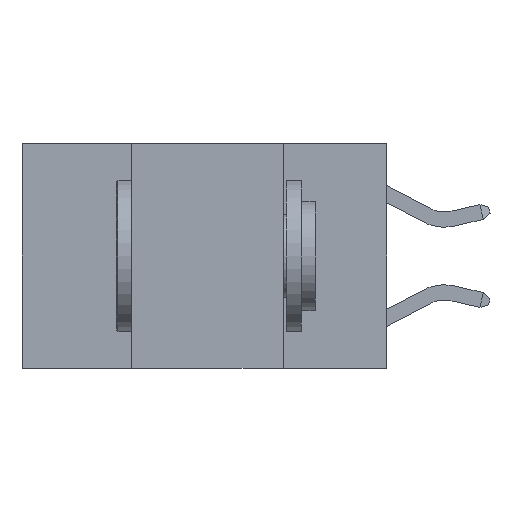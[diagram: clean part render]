
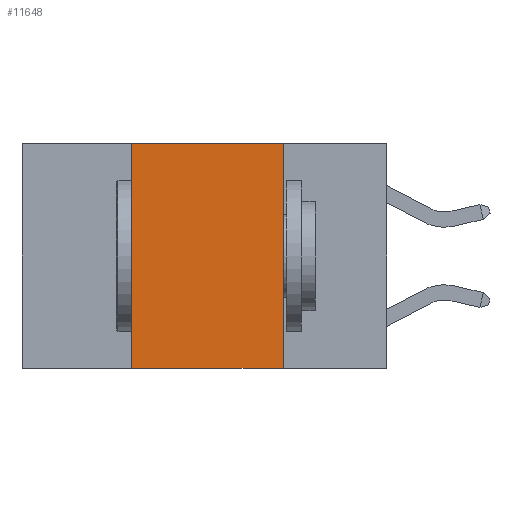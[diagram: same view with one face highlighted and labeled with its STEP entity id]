
A CAD part, left-side view. The second image highlights one B-rep face of the part: STEP entity #11648.
In plain terms, the highlighted planar face has unit normal (-1, 0, 0).
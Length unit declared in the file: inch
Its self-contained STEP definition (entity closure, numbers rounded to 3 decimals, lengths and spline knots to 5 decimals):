
#240 = AXIS2_PLACEMENT_3D ( 'NONE', #6873, #6803, #13682 ) ;
#523 = EDGE_CURVE ( 'NONE', #5476, #7634, #9982, .T. ) ;
#686 = CARTESIAN_POINT ( 'NONE',  ( 0., 0.42, 0. ) ) ;
#1471 = FACE_OUTER_BOUND ( 'NONE', #8806, .T. ) ;
#2809 = DIRECTION ( 'NONE',  ( 0., 0., -1. ) ) ;
#2942 = DIRECTION ( 'NONE',  ( 0., -1., 0. ) ) ;
#3037 = LINE ( 'NONE', #10507, #8568 ) ;
#3136 = ORIENTED_EDGE ( 'NONE', *, *, #13306, .F. ) ;
#3306 = CARTESIAN_POINT ( 'NONE',  ( 0., 0.42, 0. ) ) ;
#3372 = ORIENTED_EDGE ( 'NONE', *, *, #5863, .F. ) ;
#3624 = VECTOR ( 'NONE', #10059, 39.37008 ) ;
#3645 = CARTESIAN_POINT ( 'NONE',  ( 0., 0.42, -0.37 ) ) ;
#4118 = CARTESIAN_POINT ( 'NONE',  ( 0., 0.17, 0. ) ) ;
#4455 = VECTOR ( 'NONE', #12003, 39.37008 ) ;
#5221 = LINE ( 'NONE', #7504, #5804 ) ;
#5476 = VERTEX_POINT ( 'NONE', #686 ) ;
#5502 = LINE ( 'NONE', #3306, #4455 ) ;
#5804 = VECTOR ( 'NONE', #2942, 39.37008 ) ;
#5863 = EDGE_CURVE ( 'NONE', #7634, #10555, #3037, .T. ) ;
#5983 = PLANE ( 'NONE',  #240 ) ;
#6803 = DIRECTION ( 'NONE',  ( 1., 0., 0. ) ) ;
#6873 = CARTESIAN_POINT ( 'NONE',  ( 0., 0.6, 0. ) ) ;
#7504 = CARTESIAN_POINT ( 'NONE',  ( 0., 0.6, -0.37 ) ) ;
#7610 = EDGE_CURVE ( 'NONE', #11188, #10555, #5221, .T. ) ;
#7634 = VERTEX_POINT ( 'NONE', #4118 ) ;
#8568 = VECTOR ( 'NONE', #2809, 39.37008 ) ;
#8588 = ORIENTED_EDGE ( 'NONE', *, *, #7610, .T. ) ;
#8806 = EDGE_LOOP ( 'NONE', ( #3372, #10696, #3136, #8588 ) ) ;
#9982 = LINE ( 'NONE', #11323, #3624 ) ;
#10059 = DIRECTION ( 'NONE',  ( 0., -1., 0. ) ) ;
#10507 = CARTESIAN_POINT ( 'NONE',  ( 0., 0.17, 0. ) ) ;
#10555 = VERTEX_POINT ( 'NONE', #13312 ) ;
#10696 = ORIENTED_EDGE ( 'NONE', *, *, #523, .F. ) ;
#11188 = VERTEX_POINT ( 'NONE', #3645 ) ;
#11323 = CARTESIAN_POINT ( 'NONE',  ( 0., 0.6, 0. ) ) ;
#11648 = ADVANCED_FACE ( 'NONE', ( #1471 ), #5983, .F. ) ;
#12003 = DIRECTION ( 'NONE',  ( 0., 0., 1. ) ) ;
#13306 = EDGE_CURVE ( 'NONE', #11188, #5476, #5502, .T. ) ;
#13312 = CARTESIAN_POINT ( 'NONE',  ( 0., 0.17, -0.37 ) ) ;
#13682 = DIRECTION ( 'NONE',  ( 0., 0., -1. ) ) ;
